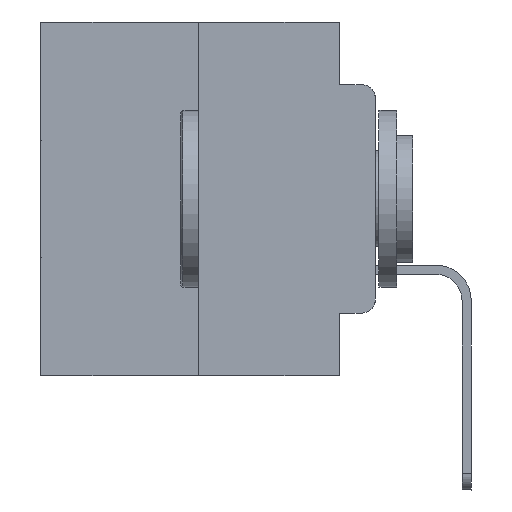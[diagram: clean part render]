
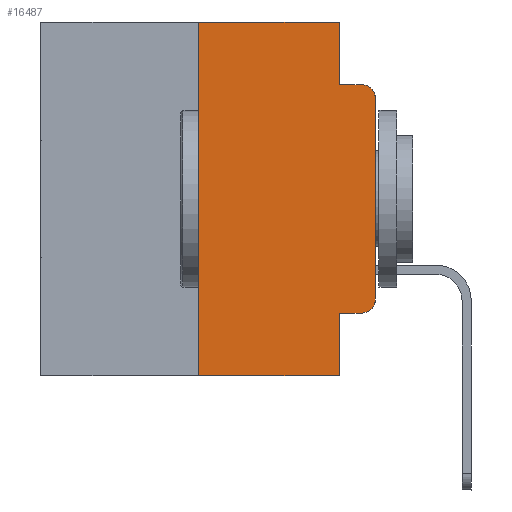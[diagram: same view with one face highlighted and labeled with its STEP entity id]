
A CAD part, left-side view. The second image highlights one B-rep face of the part: STEP entity #16487.
In plain terms, the highlighted planar face has unit normal (-1, 0, 0).
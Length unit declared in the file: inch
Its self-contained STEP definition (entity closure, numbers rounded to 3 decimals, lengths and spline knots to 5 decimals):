
#465 = CARTESIAN_POINT ( 'NONE',  ( 0., 0., -0.1085 ) ) ;
#481 = VECTOR ( 'NONE', #14927, 39.37008 ) ;
#522 = ORIENTED_EDGE ( 'NONE', *, *, #16610, .F. ) ;
#554 = VECTOR ( 'NONE', #26044, 39.37008 ) ;
#710 = VECTOR ( 'NONE', #20579, 39.37008 ) ;
#715 = VERTEX_POINT ( 'NONE', #14182 ) ;
#1019 = CARTESIAN_POINT ( 'NONE',  ( 0., 0.473, -0.5 ) ) ;
#1355 = EDGE_CURVE ( 'NONE', #3774, #6796, #3817, .T. ) ;
#2020 = ORIENTED_EDGE ( 'NONE', *, *, #18579, .F. ) ;
#2037 = CARTESIAN_POINT ( 'NONE',  ( 0., 0.25, -0.5 ) ) ;
#2640 = DIRECTION ( 'NONE',  ( -1., 0., 0. ) ) ;
#2868 = CARTESIAN_POINT ( 'NONE',  ( 0., 0.051, 0. ) ) ;
#2873 = VECTOR ( 'NONE', #16857, 39.37008 ) ;
#3054 = VERTEX_POINT ( 'NONE', #6501 ) ;
#3078 = VERTEX_POINT ( 'NONE', #26443 ) ;
#3524 = DIRECTION ( 'NONE',  ( 0., 0., -1. ) ) ;
#3774 = VERTEX_POINT ( 'NONE', #465 ) ;
#3817 = CIRCLE ( 'NONE', #13281, 0.02 ) ;
#3962 = EDGE_CURVE ( 'NONE', #23159, #4768, #4069, .T. ) ;
#4069 = LINE ( 'NONE', #17429, #26622 ) ;
#4267 = DIRECTION ( 'NONE',  ( 0., 0., 1. ) ) ;
#4433 = CARTESIAN_POINT ( 'NONE',  ( 0., 0.25, 0. ) ) ;
#4683 = CARTESIAN_POINT ( 'NONE',  ( 0., 0.02, -0.3915 ) ) ;
#4768 = VERTEX_POINT ( 'NONE', #4433 ) ;
#4939 = LINE ( 'NONE', #23735, #10324 ) ;
#5345 = ORIENTED_EDGE ( 'NONE', *, *, #6776, .F. ) ;
#5639 = PLANE ( 'NONE',  #26871 ) ;
#6501 = CARTESIAN_POINT ( 'NONE',  ( 0., 0.051, -0.5 ) ) ;
#6776 = EDGE_CURVE ( 'NONE', #17038, #3054, #9268, .T. ) ;
#6796 = VERTEX_POINT ( 'NONE', #14039 ) ;
#6904 = DIRECTION ( 'NONE',  ( 0., 0., -1. ) ) ;
#7031 = CARTESIAN_POINT ( 'NONE',  ( 0., 0.051, -0.0885 ) ) ;
#8839 = VERTEX_POINT ( 'NONE', #7031 ) ;
#9268 = LINE ( 'NONE', #2868, #710 ) ;
#9315 = EDGE_CURVE ( 'NONE', #14091, #3078, #14607, .T. ) ;
#10324 = VECTOR ( 'NONE', #19478, 39.37008 ) ;
#10346 = CARTESIAN_POINT ( 'NONE',  ( 0., 0.051, 0. ) ) ;
#10830 = LINE ( 'NONE', #1019, #21478 ) ;
#10995 = EDGE_CURVE ( 'NONE', #17038, #14091, #22378, .T. ) ;
#11276 = ORIENTED_EDGE ( 'NONE', *, *, #9315, .T. ) ;
#12290 = CARTESIAN_POINT ( 'NONE',  ( 0., 0.02, -0.1085 ) ) ;
#12293 = EDGE_CURVE ( 'NONE', #4768, #715, #4939, .T. ) ;
#12827 = DIRECTION ( 'NONE',  ( 0., -1., 0. ) ) ;
#13234 = LINE ( 'NONE', #19582, #554 ) ;
#13281 = AXIS2_PLACEMENT_3D ( 'NONE', #12290, #27696, #27894 ) ;
#14039 = CARTESIAN_POINT ( 'NONE',  ( 0., 0.02, -0.0885 ) ) ;
#14091 = VERTEX_POINT ( 'NONE', #14901 ) ;
#14182 = CARTESIAN_POINT ( 'NONE',  ( 0., 0.051, 0. ) ) ;
#14607 = CIRCLE ( 'NONE', #16556, 0.02 ) ;
#14901 = CARTESIAN_POINT ( 'NONE',  ( 0., 0.02, -0.4115 ) ) ;
#14906 = LINE ( 'NONE', #14922, #20782 ) ;
#14922 = CARTESIAN_POINT ( 'NONE',  ( 0., 0.051, -0.0885 ) ) ;
#14927 = DIRECTION ( 'NONE',  ( 0., 0., -1. ) ) ;
#15165 = EDGE_CURVE ( 'NONE', #23159, #3054, #10830, .T. ) ;
#15370 = EDGE_CURVE ( 'NONE', #3078, #3774, #13234, .T. ) ;
#16487 = ADVANCED_FACE ( 'NONE', ( #21404 ), #5639, .F. ) ;
#16556 = AXIS2_PLACEMENT_3D ( 'NONE', #4683, #2640, #6904 ) ;
#16610 = EDGE_CURVE ( 'NONE', #715, #8839, #24427, .T. ) ;
#16814 = EDGE_LOOP ( 'NONE', ( #27396, #17452, #2020, #522, #25806, #22150, #27146, #5345, #28266, #11276 ) ) ;
#16857 = DIRECTION ( 'NONE',  ( 0., -1., 0. ) ) ;
#17038 = VERTEX_POINT ( 'NONE', #20981 ) ;
#17429 = CARTESIAN_POINT ( 'NONE',  ( 0., 0.25, 0. ) ) ;
#17452 = ORIENTED_EDGE ( 'NONE', *, *, #1355, .T. ) ;
#18579 = EDGE_CURVE ( 'NONE', #8839, #6796, #14906, .T. ) ;
#19179 = CARTESIAN_POINT ( 'NONE',  ( 0., 0.051, -0.4115 ) ) ;
#19478 = DIRECTION ( 'NONE',  ( 0., -1., 0. ) ) ;
#19582 = CARTESIAN_POINT ( 'NONE',  ( 0., 0., 0. ) ) ;
#20579 = DIRECTION ( 'NONE',  ( 0., 0., -1. ) ) ;
#20782 = VECTOR ( 'NONE', #12827, 39.37008 ) ;
#20981 = CARTESIAN_POINT ( 'NONE',  ( 0., 0.051, -0.4115 ) ) ;
#21404 = FACE_OUTER_BOUND ( 'NONE', #16814, .T. ) ;
#21478 = VECTOR ( 'NONE', #27299, 39.37008 ) ;
#22150 = ORIENTED_EDGE ( 'NONE', *, *, #3962, .F. ) ;
#22378 = LINE ( 'NONE', #19179, #2873 ) ;
#23159 = VERTEX_POINT ( 'NONE', #2037 ) ;
#23178 = CARTESIAN_POINT ( 'NONE',  ( 0., 0.473, 0. ) ) ;
#23735 = CARTESIAN_POINT ( 'NONE',  ( 0., 0.473, 0. ) ) ;
#24427 = LINE ( 'NONE', #10346, #481 ) ;
#25806 = ORIENTED_EDGE ( 'NONE', *, *, #12293, .F. ) ;
#26044 = DIRECTION ( 'NONE',  ( 0., 0., 1. ) ) ;
#26443 = CARTESIAN_POINT ( 'NONE',  ( 0., 0., -0.3915 ) ) ;
#26622 = VECTOR ( 'NONE', #4267, 39.37008 ) ;
#26871 = AXIS2_PLACEMENT_3D ( 'NONE', #23178, #27291, #3524 ) ;
#27146 = ORIENTED_EDGE ( 'NONE', *, *, #15165, .T. ) ;
#27291 = DIRECTION ( 'NONE',  ( 1., 0., 0. ) ) ;
#27299 = DIRECTION ( 'NONE',  ( 0., -1., 0. ) ) ;
#27396 = ORIENTED_EDGE ( 'NONE', *, *, #15370, .T. ) ;
#27696 = DIRECTION ( 'NONE',  ( -1., 0., 0. ) ) ;
#27894 = DIRECTION ( 'NONE',  ( 0., 0., -1. ) ) ;
#28266 = ORIENTED_EDGE ( 'NONE', *, *, #10995, .T. ) ;
